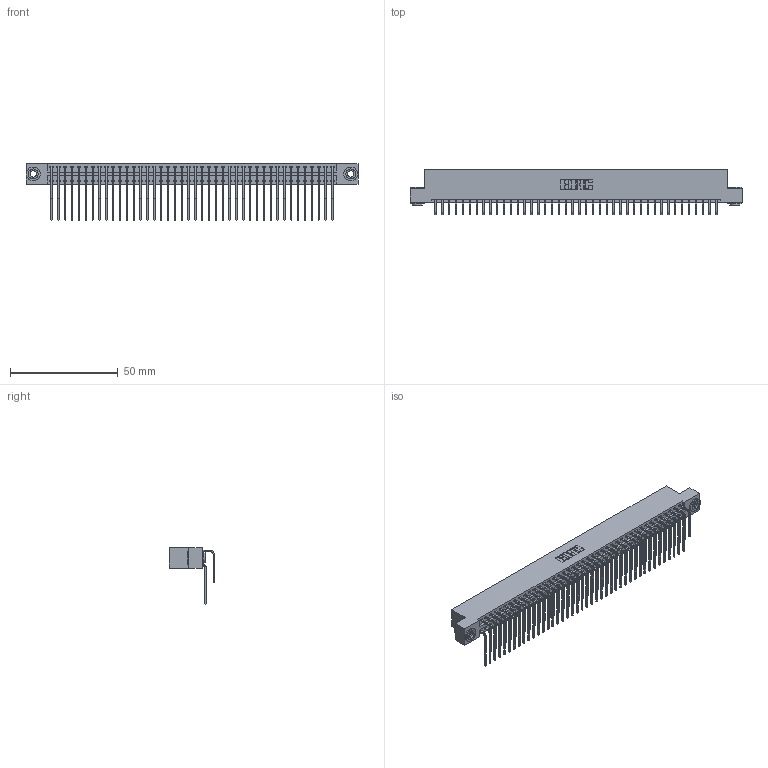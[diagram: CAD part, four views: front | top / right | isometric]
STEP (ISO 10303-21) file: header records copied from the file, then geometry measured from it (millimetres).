
FILE_DESCRIPTION (( 'STEP AP203' ), '1' );
FILE_NAME ('396-084-559-203.STEP', '2019-11-03T13:21:20', ( '' ), ( '' ), 'SwSTEP 2.0', 'SolidWorks 2016', '' );
FILE_SCHEMA (( 'CONFIG_CONTROL_DESIGN' ));
Length unit declared in the file: inch
Products named in the file (5): 396-084-559-203; 345-292-001_559 Tail - 2; 346 Part_Flush Mounting Lugs - 0.156 Dia-TH; 345-250-002_345-250-002-102; 345-292-001_558 559 Tail - 1
Assembly tree (87 placements, depth 2):
  396-084-559-203
    346 Part_Flush Mounting Lugs - 0.156 Dia-TH
    345-292-001_558 559 Tail - 1  x42
    345-292-001_559 Tail - 2  x42
    345-250-002_345-250-002-102  x2
Bounding box: 153.92 x 20.89 x 26.16 mm (x, y, z)
Volume: 15513.5 mm3; surface area: 23863.2 mm2
Topology: 87 solids, 87 shells, 4696 faces, 13929 edges, 9170 vertices
Faces by surface type: plane 3194, cylinder 1494, cone 8
Entity records: 29844 total; most frequent: CARTESIAN_POINT 4946, ORIENTED_EDGE 4822, DIRECTION 4413, EDGE_CURVE 2411, LINE 2047, VECTOR 2047, VERTEX_POINT 1602, AXIS2_PLACEMENT_3D 1183
